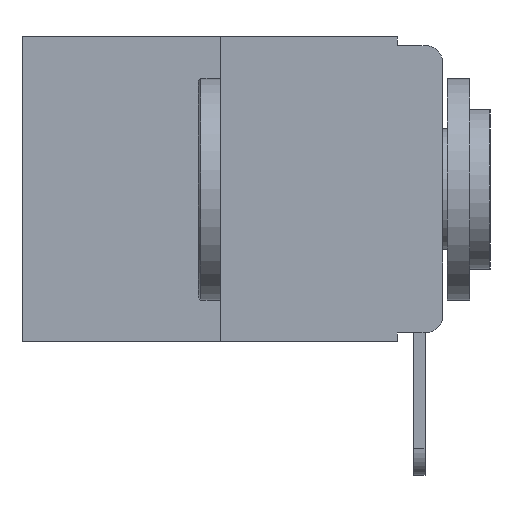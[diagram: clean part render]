
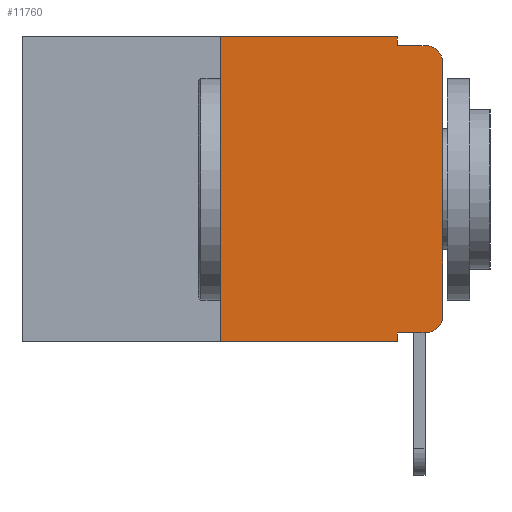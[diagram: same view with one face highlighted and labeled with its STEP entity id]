
A CAD part, left-side view. The second image highlights one B-rep face of the part: STEP entity #11760.
In plain terms, the highlighted planar face has unit normal (-1, 0, 0).
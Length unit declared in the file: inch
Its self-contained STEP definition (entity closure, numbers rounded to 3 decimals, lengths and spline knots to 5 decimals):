
#49 = EDGE_CURVE ( 'NONE', #3345, #553, #17968, .T. ) ;
#199 = CARTESIAN_POINT ( 'NONE',  ( 0., 0.051, -0.01 ) ) ;
#211 = VECTOR ( 'NONE', #19112, 39.37008 ) ;
#350 = CARTESIAN_POINT ( 'NONE',  ( 0., 0., -0.313 ) ) ;
#553 = VERTEX_POINT ( 'NONE', #199 ) ;
#675 = CIRCLE ( 'NONE', #2264, 0.02 ) ;
#1191 = DIRECTION ( 'NONE',  ( 0., 0., -1. ) ) ;
#1350 = VECTOR ( 'NONE', #8294, 39.37008 ) ;
#1419 = VERTEX_POINT ( 'NONE', #19199 ) ;
#1692 = CARTESIAN_POINT ( 'NONE',  ( 0., 0.051, -0.333 ) ) ;
#1842 = DIRECTION ( 'NONE',  ( 0., -1., 0. ) ) ;
#2264 = AXIS2_PLACEMENT_3D ( 'NONE', #7917, #10177, #10116 ) ;
#2646 = EDGE_CURVE ( 'NONE', #553, #17925, #10093, .T. ) ;
#2728 = LINE ( 'NONE', #18112, #18248 ) ;
#3345 = VERTEX_POINT ( 'NONE', #13548 ) ;
#3603 = VECTOR ( 'NONE', #1842, 39.37008 ) ;
#3626 = LINE ( 'NONE', #17746, #11798 ) ;
#3848 = CIRCLE ( 'NONE', #7269, 0.02 ) ;
#3985 = ORIENTED_EDGE ( 'NONE', *, *, #7457, .T. ) ;
#4001 = CARTESIAN_POINT ( 'NONE',  ( 0., 0.051, 0. ) ) ;
#4170 = ORIENTED_EDGE ( 'NONE', *, *, #5095, .T. ) ;
#4383 = PLANE ( 'NONE',  #5117 ) ;
#4614 = VERTEX_POINT ( 'NONE', #12617 ) ;
#4651 = DIRECTION ( 'NONE',  ( 0., 0., 1. ) ) ;
#4755 = CARTESIAN_POINT ( 'NONE',  ( 0., 0.051, -0.333 ) ) ;
#4916 = EDGE_CURVE ( 'NONE', #19631, #13475, #675, .T. ) ;
#5072 = CARTESIAN_POINT ( 'NONE',  ( 0., 0., 0. ) ) ;
#5095 = EDGE_CURVE ( 'NONE', #13799, #19631, #15740, .T. ) ;
#5117 = AXIS2_PLACEMENT_3D ( 'NONE', #5968, #10592, #1191 ) ;
#5860 = CARTESIAN_POINT ( 'NONE',  ( 0., 0.473, -0.343 ) ) ;
#5962 = EDGE_LOOP ( 'NONE', ( #15638, #3985, #12143, #16096, #16556, #9100, #13080, #19068, #4170, #16301 ) ) ;
#5968 = CARTESIAN_POINT ( 'NONE',  ( 0., 0.473, 0. ) ) ;
#6403 = CARTESIAN_POINT ( 'NONE',  ( 0., 0.02, -0.333 ) ) ;
#7269 = AXIS2_PLACEMENT_3D ( 'NONE', #8630, #18844, #10164 ) ;
#7457 = EDGE_CURVE ( 'NONE', #8303, #17925, #3848, .T. ) ;
#7917 = CARTESIAN_POINT ( 'NONE',  ( 0., 0.02, -0.313 ) ) ;
#8294 = DIRECTION ( 'NONE',  ( 0., -1., 0. ) ) ;
#8303 = VERTEX_POINT ( 'NONE', #19460 ) ;
#8380 = EDGE_CURVE ( 'NONE', #13475, #8303, #10296, .T. ) ;
#8630 = CARTESIAN_POINT ( 'NONE',  ( 0., 0.02, -0.03 ) ) ;
#8827 = DIRECTION ( 'NONE',  ( 0., 0., -1. ) ) ;
#9100 = ORIENTED_EDGE ( 'NONE', *, *, #10042, .F. ) ;
#9622 = VECTOR ( 'NONE', #15475, 39.37008 ) ;
#10042 = EDGE_CURVE ( 'NONE', #12919, #4614, #2728, .T. ) ;
#10093 = LINE ( 'NONE', #13436, #9622 ) ;
#10116 = DIRECTION ( 'NONE',  ( 0., 0., -1. ) ) ;
#10164 = DIRECTION ( 'NONE',  ( 0., 0., -1. ) ) ;
#10177 = DIRECTION ( 'NONE',  ( -1., 0., 0. ) ) ;
#10296 = LINE ( 'NONE', #5072, #13808 ) ;
#10483 = CARTESIAN_POINT ( 'NONE',  ( 0., 0.25, -0.343 ) ) ;
#10592 = DIRECTION ( 'NONE',  ( 1., 0., 0. ) ) ;
#11569 = EDGE_CURVE ( 'NONE', #4614, #3345, #13283, .T. ) ;
#11760 = ADVANCED_FACE ( 'NONE', ( #16519 ), #4383, .F. ) ;
#11798 = VECTOR ( 'NONE', #8827, 39.37008 ) ;
#12143 = ORIENTED_EDGE ( 'NONE', *, *, #2646, .F. ) ;
#12617 = CARTESIAN_POINT ( 'NONE',  ( 0., 0.25, 0. ) ) ;
#12902 = EDGE_CURVE ( 'NONE', #12919, #1419, #15806, .T. ) ;
#12919 = VERTEX_POINT ( 'NONE', #10483 ) ;
#13080 = ORIENTED_EDGE ( 'NONE', *, *, #12902, .T. ) ;
#13283 = LINE ( 'NONE', #17233, #1350 ) ;
#13436 = CARTESIAN_POINT ( 'NONE',  ( 0., 0.051, -0.01 ) ) ;
#13475 = VERTEX_POINT ( 'NONE', #350 ) ;
#13548 = CARTESIAN_POINT ( 'NONE',  ( 0., 0.051, 0. ) ) ;
#13799 = VERTEX_POINT ( 'NONE', #4755 ) ;
#13808 = VECTOR ( 'NONE', #14210, 39.37008 ) ;
#14064 = EDGE_CURVE ( 'NONE', #13799, #1419, #3626, .T. ) ;
#14210 = DIRECTION ( 'NONE',  ( 0., 0., 1. ) ) ;
#15475 = DIRECTION ( 'NONE',  ( 0., -1., 0. ) ) ;
#15638 = ORIENTED_EDGE ( 'NONE', *, *, #8380, .T. ) ;
#15740 = LINE ( 'NONE', #1692, #3603 ) ;
#15806 = LINE ( 'NONE', #5860, #211 ) ;
#15878 = DIRECTION ( 'NONE',  ( 0., 0., -1. ) ) ;
#16096 = ORIENTED_EDGE ( 'NONE', *, *, #49, .F. ) ;
#16301 = ORIENTED_EDGE ( 'NONE', *, *, #4916, .T. ) ;
#16519 = FACE_OUTER_BOUND ( 'NONE', #5962, .T. ) ;
#16556 = ORIENTED_EDGE ( 'NONE', *, *, #11569, .F. ) ;
#16627 = CARTESIAN_POINT ( 'NONE',  ( 0., 0.02, -0.01 ) ) ;
#17233 = CARTESIAN_POINT ( 'NONE',  ( 0., 0.473, 0. ) ) ;
#17571 = VECTOR ( 'NONE', #15878, 39.37008 ) ;
#17746 = CARTESIAN_POINT ( 'NONE',  ( 0., 0.051, 0. ) ) ;
#17925 = VERTEX_POINT ( 'NONE', #16627 ) ;
#17968 = LINE ( 'NONE', #4001, #17571 ) ;
#18112 = CARTESIAN_POINT ( 'NONE',  ( 0., 0.25, 0. ) ) ;
#18248 = VECTOR ( 'NONE', #4651, 39.37008 ) ;
#18844 = DIRECTION ( 'NONE',  ( -1., 0., 0. ) ) ;
#19068 = ORIENTED_EDGE ( 'NONE', *, *, #14064, .F. ) ;
#19112 = DIRECTION ( 'NONE',  ( 0., -1., 0. ) ) ;
#19199 = CARTESIAN_POINT ( 'NONE',  ( 0., 0.051, -0.343 ) ) ;
#19460 = CARTESIAN_POINT ( 'NONE',  ( 0., 0., -0.03 ) ) ;
#19631 = VERTEX_POINT ( 'NONE', #6403 ) ;
